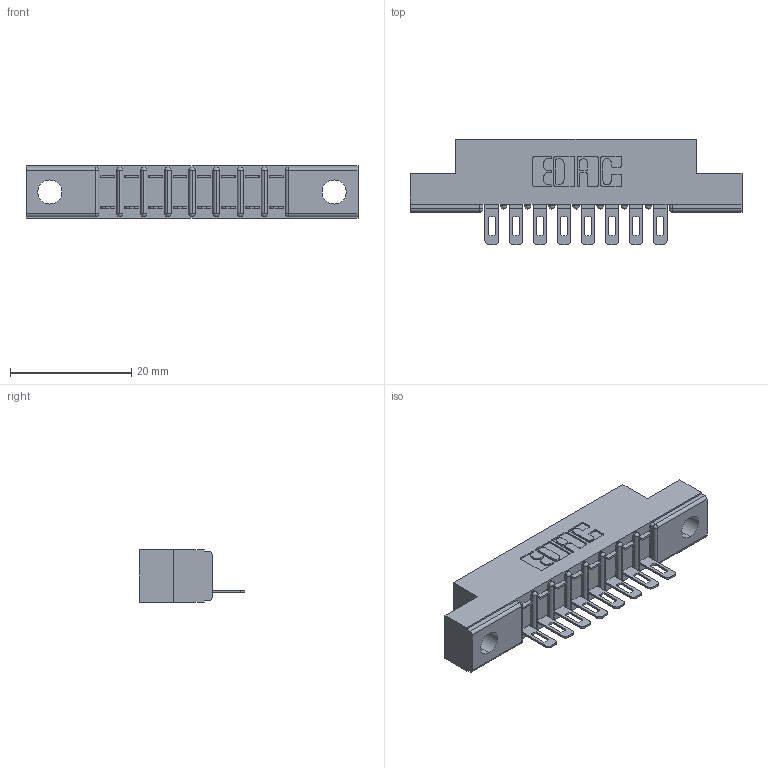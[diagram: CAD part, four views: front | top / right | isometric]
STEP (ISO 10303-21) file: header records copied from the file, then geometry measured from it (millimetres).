
FILE_DESCRIPTION (( 'STEP AP203' ), '1' );
FILE_NAME ('357-008-501-104.STEP', '2019-09-16T17:35:33', ( '' ), ( '' ), 'SwSTEP 2.0', 'SolidWorks 2016', '' );
FILE_SCHEMA (( 'CONFIG_CONTROL_DESIGN' ));
Length unit declared in the file: inch
Products named in the file (3): 307 Part_.156 Dia Mounting Holes; 357-008-501-104; 307-290-002_501
Assembly tree (9 placements, depth 2):
  357-008-501-104
    307 Part_.156 Dia Mounting Holes
    307-290-002_501  x8
Bounding box: 54.71 x 17.42 x 8.71 mm (x, y, z)
Volume: 3505.6 mm3; surface area: 5542.3 mm2
Topology: 9 solids, 9 shells, 749 faces, 2263 edges, 1482 vertices
Faces by surface type: plane 436, cylinder 295, sphere 18
Entity records: 12262 total; most frequent: CARTESIAN_POINT 2066, ORIENTED_EDGE 2054, DIRECTION 2019, EDGE_CURVE 1027, LINE 773, VECTOR 773, VERTEX_POINT 670, AXIS2_PLACEMENT_3D 623
